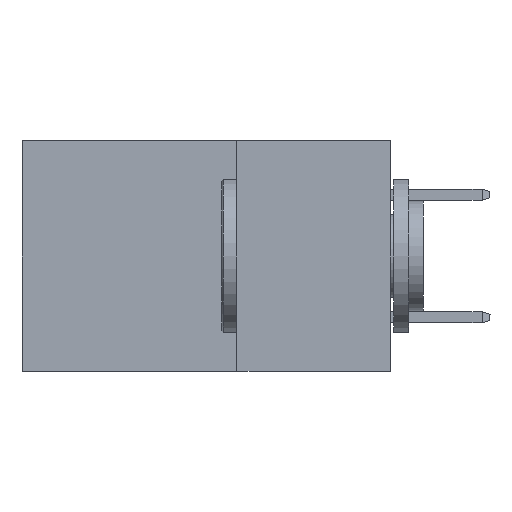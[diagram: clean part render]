
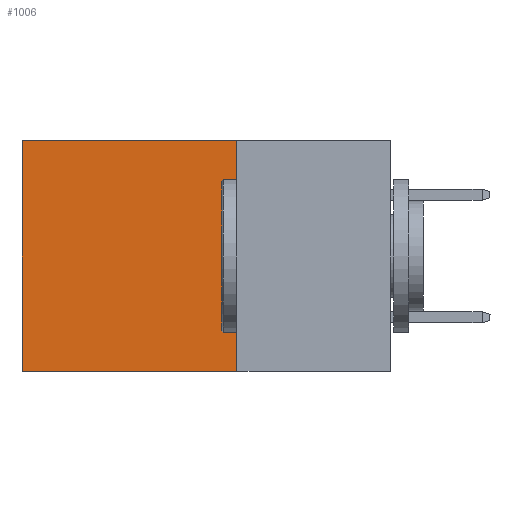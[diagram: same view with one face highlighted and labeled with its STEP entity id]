
A CAD part, left-side view. The second image highlights one B-rep face of the part: STEP entity #1006.
In plain terms, the highlighted planar face has unit normal (-1, 0, 0).
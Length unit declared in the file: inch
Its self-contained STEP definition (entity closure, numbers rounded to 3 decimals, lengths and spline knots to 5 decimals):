
#101 = VECTOR ( 'NONE', #15731, 39.37008 ) ;
#481 = EDGE_CURVE ( 'NONE', #6498, #7727, #9474, .T. ) ;
#1006 = ADVANCED_FACE ( 'NONE', ( #8055 ), #7404, .F. ) ;
#2258 = DIRECTION ( 'NONE',  ( 1., 0., 0. ) ) ;
#2633 = CARTESIAN_POINT ( 'NONE',  ( 0.2875, 0.25, -0.375 ) ) ;
#3634 = LINE ( 'NONE', #15617, #101 ) ;
#4351 = CARTESIAN_POINT ( 'NONE',  ( 0.2875, 0.6, -0.375 ) ) ;
#5701 = ORIENTED_EDGE ( 'NONE', *, *, #7025, .F. ) ;
#5837 = VECTOR ( 'NONE', #6503, 39.37008 ) ;
#6498 = VERTEX_POINT ( 'NONE', #8907 ) ;
#6503 = DIRECTION ( 'NONE',  ( 0., 0., -1. ) ) ;
#6610 = LINE ( 'NONE', #14743, #8240 ) ;
#6921 = ORIENTED_EDGE ( 'NONE', *, *, #481, .T. ) ;
#7025 = EDGE_CURVE ( 'NONE', #11581, #9370, #12209, .T. ) ;
#7404 = PLANE ( 'NONE',  #13713 ) ;
#7727 = VERTEX_POINT ( 'NONE', #4351 ) ;
#7845 = EDGE_CURVE ( 'NONE', #9370, #7727, #6610, .T. ) ;
#8055 = FACE_OUTER_BOUND ( 'NONE', #13746, .T. ) ;
#8240 = VECTOR ( 'NONE', #12215, 39.37008 ) ;
#8907 = CARTESIAN_POINT ( 'NONE',  ( 0.2875, 0.6, 0. ) ) ;
#9370 = VERTEX_POINT ( 'NONE', #9513 ) ;
#9474 = LINE ( 'NONE', #10213, #13831 ) ;
#9513 = CARTESIAN_POINT ( 'NONE',  ( 0.2875, 0.25, -0.375 ) ) ;
#10056 = DIRECTION ( 'NONE',  ( 0., 0., -1. ) ) ;
#10213 = CARTESIAN_POINT ( 'NONE',  ( 0.2875, 0.6, -0.375 ) ) ;
#11581 = VERTEX_POINT ( 'NONE', #15938 ) ;
#12209 = LINE ( 'NONE', #2633, #5837 ) ;
#12215 = DIRECTION ( 'NONE',  ( 0., 1., 0. ) ) ;
#12388 = DIRECTION ( 'NONE',  ( 0., 0., -1. ) ) ;
#12894 = ORIENTED_EDGE ( 'NONE', *, *, #7845, .F. ) ;
#13713 = AXIS2_PLACEMENT_3D ( 'NONE', #15086, #2258, #12388 ) ;
#13746 = EDGE_LOOP ( 'NONE', ( #6921, #12894, #5701, #13936 ) ) ;
#13831 = VECTOR ( 'NONE', #10056, 39.37008 ) ;
#13936 = ORIENTED_EDGE ( 'NONE', *, *, #15540, .T. ) ;
#14743 = CARTESIAN_POINT ( 'NONE',  ( 0.2875, 0.25, -0.375 ) ) ;
#15086 = CARTESIAN_POINT ( 'NONE',  ( 0.2875, 0.25, -0.375 ) ) ;
#15540 = EDGE_CURVE ( 'NONE', #11581, #6498, #3634, .T. ) ;
#15617 = CARTESIAN_POINT ( 'NONE',  ( 0.2875, 0.25, 0. ) ) ;
#15731 = DIRECTION ( 'NONE',  ( 0., 1., 0. ) ) ;
#15938 = CARTESIAN_POINT ( 'NONE',  ( 0.2875, 0.25, 0. ) ) ;
